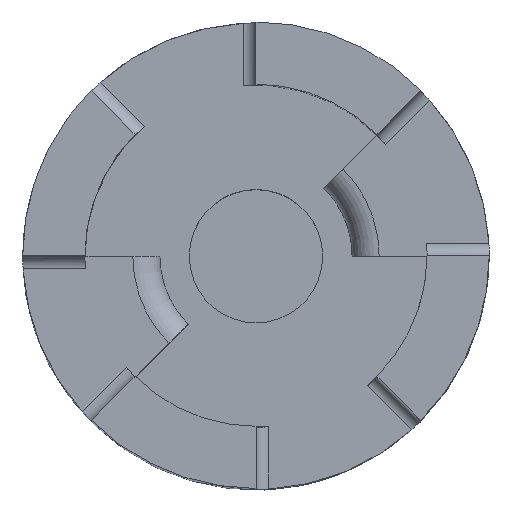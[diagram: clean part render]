
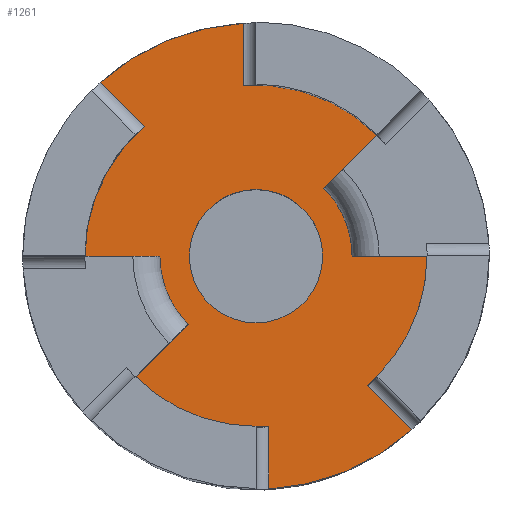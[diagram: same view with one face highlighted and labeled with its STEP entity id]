
A CAD part, top view. The second image highlights one B-rep face of the part: STEP entity #1261.
In plain terms, the highlighted planar face has unit normal (0, 0, 1).
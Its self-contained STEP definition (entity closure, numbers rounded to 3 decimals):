
#50=FACE_BOUND('',#249,.T.);
#118=PLANE('',#1365);
#179=FACE_OUTER_BOUND('',#248,.T.);
#248=EDGE_LOOP('',(#1081,#1082,#1083,#1084,#1085,#1086,#1087,#1088,#1089,
#1090,#1091,#1092,#1093,#1094,#1095,#1096));
#249=EDGE_LOOP('',(#1097));
#272=LINE('',#1695,#360);
#279=LINE('',#1724,#367);
#332=LINE('',#2712,#420);
#335=LINE('',#2730,#423);
#337=LINE('',#2736,#425);
#338=LINE('',#2740,#426);
#339=LINE('',#2742,#427);
#340=LINE('',#2746,#428);
#360=VECTOR('',#1418,10.);
#367=VECTOR('',#1445,10.);
#420=VECTOR('',#1584,10.);
#423=VECTOR('',#1591,10.);
#425=VECTOR('',#1597,10.);
#426=VECTOR('',#1602,10.);
#427=VECTOR('',#1603,10.);
#428=VECTOR('',#1606,10.);
#445=CIRCLE('',#1302,3.125);
#462=CIRCLE('',#1332,10.922);
#470=CIRCLE('',#1340,10.922);
#482=CIRCLE('',#1366,8.01);
#483=CIRCLE('',#1367,4.5);
#484=CIRCLE('',#1368,8.01);
#485=CIRCLE('',#1369,8.01);
#486=CIRCLE('',#1370,4.5);
#487=CIRCLE('',#1371,8.01);
#492=VERTEX_POINT('',#1675);
#499=VERTEX_POINT('',#1692);
#500=VERTEX_POINT('',#1694);
#511=VERTEX_POINT('',#1721);
#512=VERTEX_POINT('',#1723);
#532=VERTEX_POINT('',#1851);
#533=VERTEX_POINT('',#1862);
#548=VERTEX_POINT('',#1903);
#549=VERTEX_POINT('',#1914);
#601=VERTEX_POINT('',#2699);
#605=VERTEX_POINT('',#2719);
#606=VERTEX_POINT('',#2733);
#607=VERTEX_POINT('',#2735);
#608=VERTEX_POINT('',#2738);
#609=VERTEX_POINT('',#2741);
#610=VERTEX_POINT('',#2743);
#611=VERTEX_POINT('',#2745);
#619=EDGE_CURVE('',#492,#492,#445,.T.);
#628=EDGE_CURVE('',#500,#499,#272,.T.);
#642=EDGE_CURVE('',#512,#511,#279,.T.);
#671=EDGE_CURVE('',#533,#532,#462,.F.);
#689=EDGE_CURVE('',#549,#548,#470,.F.);
#772=EDGE_CURVE('',#549,#601,#332,.T.);
#776=EDGE_CURVE('',#605,#548,#335,.T.);
#778=EDGE_CURVE('',#605,#606,#482,.T.);
#779=EDGE_CURVE('',#606,#607,#337,.T.);
#780=EDGE_CURVE('',#512,#607,#483,.T.);
#781=EDGE_CURVE('',#511,#608,#484,.T.);
#782=EDGE_CURVE('',#533,#608,#338,.T.);
#783=EDGE_CURVE('',#609,#532,#339,.T.);
#784=EDGE_CURVE('',#609,#610,#485,.T.);
#785=EDGE_CURVE('',#610,#611,#340,.T.);
#786=EDGE_CURVE('',#500,#611,#486,.T.);
#787=EDGE_CURVE('',#499,#601,#487,.T.);
#1081=ORIENTED_EDGE('',*,*,#772,.F.);
#1082=ORIENTED_EDGE('',*,*,#689,.T.);
#1083=ORIENTED_EDGE('',*,*,#776,.F.);
#1084=ORIENTED_EDGE('',*,*,#778,.T.);
#1085=ORIENTED_EDGE('',*,*,#779,.T.);
#1086=ORIENTED_EDGE('',*,*,#780,.F.);
#1087=ORIENTED_EDGE('',*,*,#642,.T.);
#1088=ORIENTED_EDGE('',*,*,#781,.T.);
#1089=ORIENTED_EDGE('',*,*,#782,.F.);
#1090=ORIENTED_EDGE('',*,*,#671,.T.);
#1091=ORIENTED_EDGE('',*,*,#783,.F.);
#1092=ORIENTED_EDGE('',*,*,#784,.T.);
#1093=ORIENTED_EDGE('',*,*,#785,.T.);
#1094=ORIENTED_EDGE('',*,*,#786,.F.);
#1095=ORIENTED_EDGE('',*,*,#628,.T.);
#1096=ORIENTED_EDGE('',*,*,#787,.T.);
#1097=ORIENTED_EDGE('',*,*,#619,.T.);
#1261=ADVANCED_FACE('',(#179,#50),#118,.T.);
#1302=AXIS2_PLACEMENT_3D('',#1676,#1399,#1400);
#1332=AXIS2_PLACEMENT_3D('',#1863,#1485,#1486);
#1340=AXIS2_PLACEMENT_3D('',#1915,#1509,#1510);
#1365=AXIS2_PLACEMENT_3D('',#2732,#1593,#1594);
#1366=AXIS2_PLACEMENT_3D('',#2734,#1595,#1596);
#1367=AXIS2_PLACEMENT_3D('',#2737,#1598,#1599);
#1368=AXIS2_PLACEMENT_3D('',#2739,#1600,#1601);
#1369=AXIS2_PLACEMENT_3D('',#2744,#1604,#1605);
#1370=AXIS2_PLACEMENT_3D('',#2747,#1607,#1608);
#1371=AXIS2_PLACEMENT_3D('',#2748,#1609,#1610);
#1399=DIRECTION('center_axis',(0.,0.,-1.));
#1400=DIRECTION('ref_axis',(1.,0.,0.));
#1418=DIRECTION('',(0.707,0.707,0.));
#1445=DIRECTION('',(-0.707,-0.707,0.));
#1485=DIRECTION('center_axis',(0.,0.,-1.));
#1486=DIRECTION('ref_axis',(1.,0.,0.));
#1509=DIRECTION('center_axis',(0.,0.,-1.));
#1510=DIRECTION('ref_axis',(1.,0.,0.));
#1584=DIRECTION('',(0.,-1.,0.));
#1591=DIRECTION('',(-0.707,0.707,0.));
#1593=DIRECTION('center_axis',(0.,0.,1.));
#1594=DIRECTION('ref_axis',(1.,0.,0.));
#1595=DIRECTION('center_axis',(0.,0.,1.));
#1596=DIRECTION('ref_axis',(0.707,-0.707,0.));
#1597=DIRECTION('',(1.,0.,0.));
#1598=DIRECTION('center_axis',(0.,0.,-1.));
#1599=DIRECTION('ref_axis',(1.,0.,0.));
#1600=DIRECTION('center_axis',(0.,0.,1.));
#1601=DIRECTION('ref_axis',(0.707,-0.707,0.));
#1602=DIRECTION('',(0.,1.,0.));
#1603=DIRECTION('',(0.707,-0.707,0.));
#1604=DIRECTION('center_axis',(0.,0.,1.));
#1605=DIRECTION('ref_axis',(-0.707,0.707,0.));
#1606=DIRECTION('',(-1.,0.,0.));
#1607=DIRECTION('center_axis',(0.,0.,-1.));
#1608=DIRECTION('ref_axis',(1.,0.,0.));
#1609=DIRECTION('center_axis',(0.,0.,1.));
#1610=DIRECTION('ref_axis',(-0.707,0.707,0.));
#1675=CARTESIAN_POINT('',(-3.125,0.,2.54));
#1676=CARTESIAN_POINT('Origin',(0.,0.,2.54));
#1692=CARTESIAN_POINT('',(5.664,5.664,2.54));
#1694=CARTESIAN_POINT('',(3.182,3.182,2.54));
#1695=CARTESIAN_POINT('',(2.832,2.832,2.54));
#1721=CARTESIAN_POINT('',(-5.664,-5.664,2.54));
#1723=CARTESIAN_POINT('',(-3.182,-3.182,2.54));
#1724=CARTESIAN_POINT('',(-2.832,-2.832,2.54));
#1851=CARTESIAN_POINT('',(7.287,-8.136,2.54));
#1862=CARTESIAN_POINT('',(0.6,-10.906,2.54));
#1863=CARTESIAN_POINT('Origin',(0.,0.,2.54));
#1903=CARTESIAN_POINT('',(-7.287,8.136,2.54));
#1914=CARTESIAN_POINT('',(-0.6,10.906,2.54));
#1915=CARTESIAN_POINT('Origin',(0.,0.,2.54));
#2699=CARTESIAN_POINT('',(-0.6,7.987,2.54));
#2712=CARTESIAN_POINT('',(-0.6,5.08,2.54));
#2719=CARTESIAN_POINT('',(-5.224,6.072,2.54));
#2730=CARTESIAN_POINT('',(-2.408,3.256,2.54));
#2732=CARTESIAN_POINT('Origin',(0.,0.,
2.54));
#2733=CARTESIAN_POINT('',(-8.01,0.,2.54));
#2734=CARTESIAN_POINT('Origin',(0.,0.,
2.54));
#2735=CARTESIAN_POINT('',(-4.5,0.,2.54));
#2736=CARTESIAN_POINT('',(-1.594,0.,2.54));
#2737=CARTESIAN_POINT('Origin',(0.,0.,2.54));
#2738=CARTESIAN_POINT('',(0.6,-7.987,2.54));
#2739=CARTESIAN_POINT('Origin',(0.,0.,
2.54));
#2740=CARTESIAN_POINT('',(0.6,-5.08,2.54));
#2741=CARTESIAN_POINT('',(5.224,-6.072,2.54));
#2742=CARTESIAN_POINT('',(2.408,-3.256,2.54));
#2743=CARTESIAN_POINT('',(8.01,0.,2.54));
#2744=CARTESIAN_POINT('Origin',(0.,0.,
2.54));
#2745=CARTESIAN_POINT('',(4.5,0.,2.54));
#2746=CARTESIAN_POINT('',(1.594,0.,2.54));
#2747=CARTESIAN_POINT('Origin',(0.,0.,2.54));
#2748=CARTESIAN_POINT('Origin',(0.,0.,
2.54));
